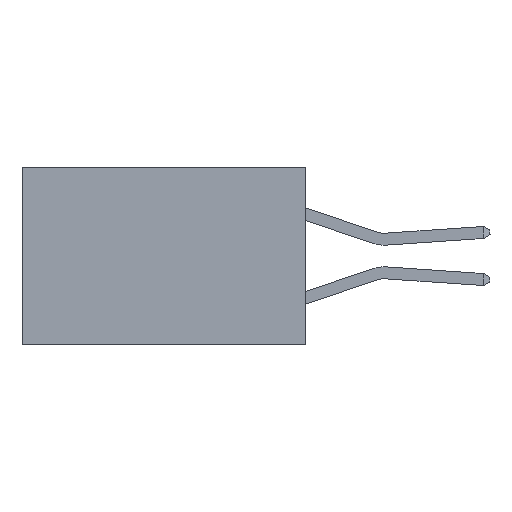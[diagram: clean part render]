
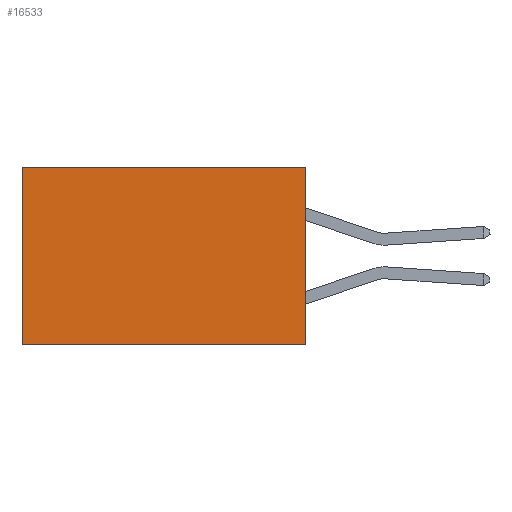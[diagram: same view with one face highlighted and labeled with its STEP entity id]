
A CAD part, left-side view. The second image highlights one B-rep face of the part: STEP entity #16533.
In plain terms, the highlighted planar face has unit normal (-1, 0, 0).
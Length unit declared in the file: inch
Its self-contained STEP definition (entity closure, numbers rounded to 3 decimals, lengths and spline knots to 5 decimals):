
#385 = CARTESIAN_POINT ( 'NONE',  ( 0.277, 0., -0.37 ) ) ;
#489 = VERTEX_POINT ( 'NONE', #3722 ) ;
#904 = EDGE_CURVE ( 'NONE', #12514, #7344, #10638, .T. ) ;
#1219 = PLANE ( 'NONE',  #17099 ) ;
#1785 = VECTOR ( 'NONE', #15719, 39.37008 ) ;
#1796 = DIRECTION ( 'NONE',  ( 0., 0., -1. ) ) ;
#2325 = LINE ( 'NONE', #8373, #9352 ) ;
#2462 = DIRECTION ( 'NONE',  ( 0., 1., 0. ) ) ;
#2663 = CARTESIAN_POINT ( 'NONE',  ( 0.277, 0., -0.37 ) ) ;
#2889 = ORIENTED_EDGE ( 'NONE', *, *, #6630, .F. ) ;
#3722 = CARTESIAN_POINT ( 'NONE',  ( 0.277, 0., -0.37 ) ) ;
#4075 = DIRECTION ( 'NONE',  ( 1., 0., 0. ) ) ;
#4180 = CARTESIAN_POINT ( 'NONE',  ( 0.277, 0.59, -0.37 ) ) ;
#5555 = LINE ( 'NONE', #16225, #1785 ) ;
#6005 = VECTOR ( 'NONE', #1796, 39.37008 ) ;
#6630 = EDGE_CURVE ( 'NONE', #489, #12958, #5555, .T. ) ;
#6957 = FACE_OUTER_BOUND ( 'NONE', #10600, .T. ) ;
#7344 = VERTEX_POINT ( 'NONE', #7738 ) ;
#7738 = CARTESIAN_POINT ( 'NONE',  ( 0.277, 0.59, 0. ) ) ;
#8373 = CARTESIAN_POINT ( 'NONE',  ( 0.277, 0.59, -0.37 ) ) ;
#9352 = VECTOR ( 'NONE', #9779, 39.37008 ) ;
#9779 = DIRECTION ( 'NONE',  ( 0., 0., -1. ) ) ;
#10600 = EDGE_LOOP ( 'NONE', ( #17470, #2889, #16989, #15825 ) ) ;
#10638 = LINE ( 'NONE', #16872, #17503 ) ;
#11772 = EDGE_CURVE ( 'NONE', #12514, #489, #17045, .T. ) ;
#12514 = VERTEX_POINT ( 'NONE', #14385 ) ;
#12958 = VERTEX_POINT ( 'NONE', #4180 ) ;
#13798 = DIRECTION ( 'NONE',  ( 0., 0., -1. ) ) ;
#14385 = CARTESIAN_POINT ( 'NONE',  ( 0.277, 0., 0. ) ) ;
#15719 = DIRECTION ( 'NONE',  ( 0., 1., 0. ) ) ;
#15825 = ORIENTED_EDGE ( 'NONE', *, *, #904, .T. ) ;
#15905 = EDGE_CURVE ( 'NONE', #7344, #12958, #2325, .T. ) ;
#16225 = CARTESIAN_POINT ( 'NONE',  ( 0.277, 0., -0.37 ) ) ;
#16533 = ADVANCED_FACE ( 'NONE', ( #6957 ), #1219, .F. ) ;
#16872 = CARTESIAN_POINT ( 'NONE',  ( 0.277, 0., 0. ) ) ;
#16989 = ORIENTED_EDGE ( 'NONE', *, *, #11772, .F. ) ;
#17045 = LINE ( 'NONE', #385, #6005 ) ;
#17099 = AXIS2_PLACEMENT_3D ( 'NONE', #2663, #4075, #13798 ) ;
#17470 = ORIENTED_EDGE ( 'NONE', *, *, #15905, .T. ) ;
#17503 = VECTOR ( 'NONE', #2462, 39.37008 ) ;
